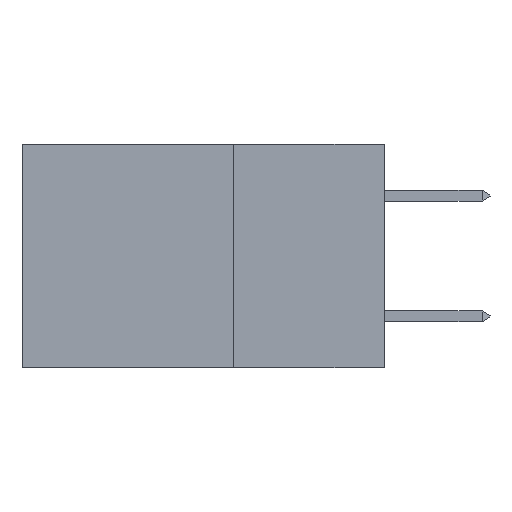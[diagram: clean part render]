
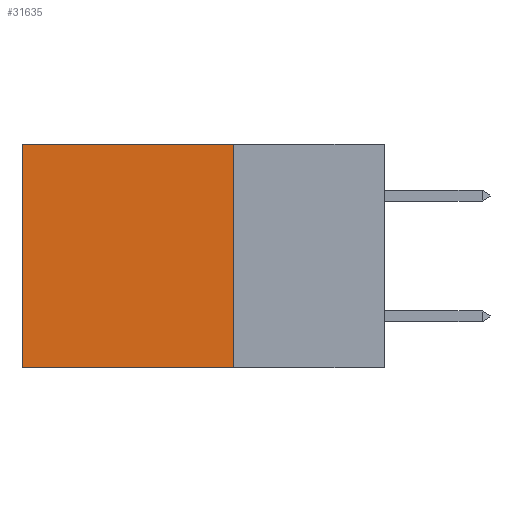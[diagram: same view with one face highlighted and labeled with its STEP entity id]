
A CAD part, left-side view. The second image highlights one B-rep face of the part: STEP entity #31635.
In plain terms, the highlighted planar face has unit normal (-1, 0, 0).
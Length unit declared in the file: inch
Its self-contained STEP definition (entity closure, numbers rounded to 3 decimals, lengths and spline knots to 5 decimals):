
#539 = CARTESIAN_POINT ( 'NONE',  ( 0.2875, 0.25, 0. ) ) ;
#2885 = LINE ( 'NONE', #26592, #11581 ) ;
#3046 = EDGE_CURVE ( 'NONE', #7044, #25802, #3270, .T. ) ;
#3270 = LINE ( 'NONE', #18135, #22871 ) ;
#3548 = AXIS2_PLACEMENT_3D ( 'NONE', #539, #29810, #10345 ) ;
#3624 = PLANE ( 'NONE',  #3548 ) ;
#7044 = VERTEX_POINT ( 'NONE', #30419 ) ;
#7443 = LINE ( 'NONE', #35791, #36782 ) ;
#10345 = DIRECTION ( 'NONE',  ( 0., 0., -1. ) ) ;
#11581 = VECTOR ( 'NONE', #26214, 39.37008 ) ;
#13310 = CARTESIAN_POINT ( 'NONE',  ( 0.2875, 0.6, 0. ) ) ;
#14515 = EDGE_LOOP ( 'NONE', ( #28535, #30925, #20662, #30216 ) ) ;
#16014 = EDGE_CURVE ( 'NONE', #25163, #7044, #2885, .T. ) ;
#16360 = EDGE_CURVE ( 'NONE', #25177, #25802, #27924, .T. ) ;
#17170 = CARTESIAN_POINT ( 'NONE',  ( 0.2875, 0.6, 0. ) ) ;
#18135 = CARTESIAN_POINT ( 'NONE',  ( 0.2875, 0.25, -0.37 ) ) ;
#19011 = FACE_OUTER_BOUND ( 'NONE', #14515, .T. ) ;
#19193 = DIRECTION ( 'NONE',  ( 0., 1., 0. ) ) ;
#20256 = DIRECTION ( 'NONE',  ( 0., 1., 0. ) ) ;
#20662 = ORIENTED_EDGE ( 'NONE', *, *, #16014, .F. ) ;
#22871 = VECTOR ( 'NONE', #20256, 39.37008 ) ;
#24699 = CARTESIAN_POINT ( 'NONE',  ( 0.2875, 0.25, 0. ) ) ;
#25040 = DIRECTION ( 'NONE',  ( 0., 0., -1. ) ) ;
#25163 = VERTEX_POINT ( 'NONE', #24699 ) ;
#25177 = VERTEX_POINT ( 'NONE', #17170 ) ;
#25802 = VERTEX_POINT ( 'NONE', #35346 ) ;
#26214 = DIRECTION ( 'NONE',  ( 0., 0., -1. ) ) ;
#26592 = CARTESIAN_POINT ( 'NONE',  ( 0.2875, 0.25, 0. ) ) ;
#27924 = LINE ( 'NONE', #13310, #36187 ) ;
#28535 = ORIENTED_EDGE ( 'NONE', *, *, #16360, .T. ) ;
#29810 = DIRECTION ( 'NONE',  ( 1., 0., 0. ) ) ;
#30216 = ORIENTED_EDGE ( 'NONE', *, *, #31665, .T. ) ;
#30419 = CARTESIAN_POINT ( 'NONE',  ( 0.2875, 0.25, -0.37 ) ) ;
#30925 = ORIENTED_EDGE ( 'NONE', *, *, #3046, .F. ) ;
#31635 = ADVANCED_FACE ( 'NONE', ( #19011 ), #3624, .F. ) ;
#31665 = EDGE_CURVE ( 'NONE', #25163, #25177, #7443, .T. ) ;
#35346 = CARTESIAN_POINT ( 'NONE',  ( 0.2875, 0.6, -0.37 ) ) ;
#35791 = CARTESIAN_POINT ( 'NONE',  ( 0.2875, 0.25, 0. ) ) ;
#36187 = VECTOR ( 'NONE', #25040, 39.37008 ) ;
#36782 = VECTOR ( 'NONE', #19193, 39.37008 ) ;
